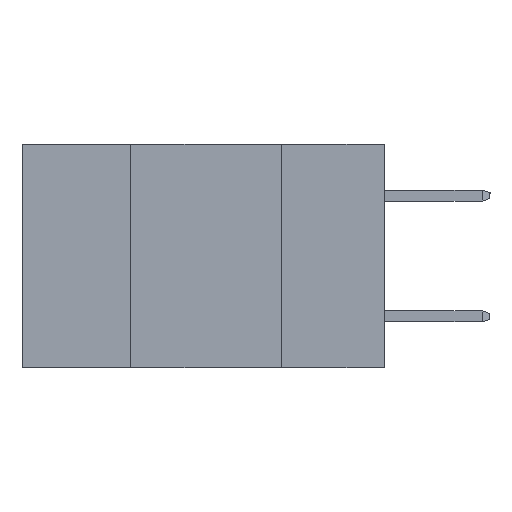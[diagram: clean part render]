
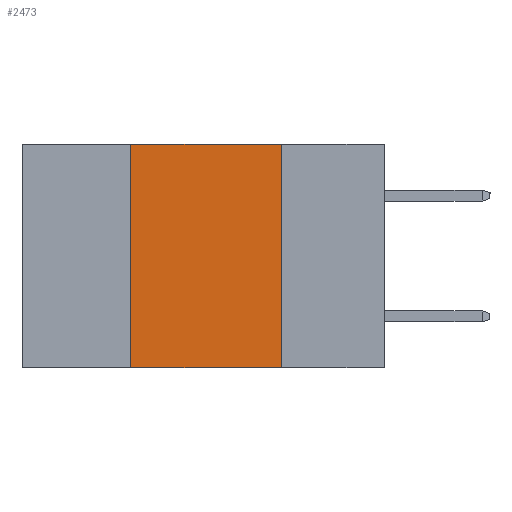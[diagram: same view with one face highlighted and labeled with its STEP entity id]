
A CAD part, left-side view. The second image highlights one B-rep face of the part: STEP entity #2473.
In plain terms, the highlighted planar face has unit normal (-1, 0, 0).
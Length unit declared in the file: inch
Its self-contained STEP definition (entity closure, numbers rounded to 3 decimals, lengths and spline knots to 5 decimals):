
#1633 = VECTOR ( 'NONE', #8139, 39.37008 ) ;
#2008 = ORIENTED_EDGE ( 'NONE', *, *, #7815, .F. ) ;
#2473 = ADVANCED_FACE ( 'NONE', ( #11334 ), #6077, .F. ) ;
#3653 = VECTOR ( 'NONE', #16933, 39.37008 ) ;
#3939 = ORIENTED_EDGE ( 'NONE', *, *, #19292, .F. ) ;
#4271 = EDGE_CURVE ( 'NONE', #17961, #8135, #6595, .T. ) ;
#4904 = EDGE_LOOP ( 'NONE', ( #3939, #17289, #2008, #9329 ) ) ;
#6077 = PLANE ( 'NONE',  #19034 ) ;
#6259 = VECTOR ( 'NONE', #8287, 39.37008 ) ;
#6595 = LINE ( 'NONE', #10071, #6259 ) ;
#6774 = LINE ( 'NONE', #18643, #1633 ) ;
#7815 = EDGE_CURVE ( 'NONE', #17961, #15126, #6774, .T. ) ;
#8135 = VERTEX_POINT ( 'NONE', #19822 ) ;
#8139 = DIRECTION ( 'NONE',  ( 0., 0., 1. ) ) ;
#8287 = DIRECTION ( 'NONE',  ( 0., -1., 0. ) ) ;
#9329 = ORIENTED_EDGE ( 'NONE', *, *, #4271, .T. ) ;
#9493 = VECTOR ( 'NONE', #20148, 39.37008 ) ;
#10071 = CARTESIAN_POINT ( 'NONE',  ( 0., 0.6, -0.37 ) ) ;
#11334 = FACE_OUTER_BOUND ( 'NONE', #4904, .T. ) ;
#11854 = VERTEX_POINT ( 'NONE', #12383 ) ;
#11885 = LINE ( 'NONE', #22098, #3653 ) ;
#12383 = CARTESIAN_POINT ( 'NONE',  ( 0., 0.17, 0. ) ) ;
#13191 = CARTESIAN_POINT ( 'NONE',  ( 0., 0.17, -0.37 ) ) ;
#13498 = EDGE_CURVE ( 'NONE', #15126, #11854, #11885, .T. ) ;
#13590 = CARTESIAN_POINT ( 'NONE',  ( 0., 0.42, -0.37 ) ) ;
#15017 = DIRECTION ( 'NONE',  ( 0., 0., -1. ) ) ;
#15126 = VERTEX_POINT ( 'NONE', #15603 ) ;
#15603 = CARTESIAN_POINT ( 'NONE',  ( 0., 0.42, 0. ) ) ;
#16480 = CARTESIAN_POINT ( 'NONE',  ( 0., 0.6, 0. ) ) ;
#16933 = DIRECTION ( 'NONE',  ( 0., -1., 0. ) ) ;
#17289 = ORIENTED_EDGE ( 'NONE', *, *, #13498, .F. ) ;
#17961 = VERTEX_POINT ( 'NONE', #13590 ) ;
#18463 = LINE ( 'NONE', #13191, #9493 ) ;
#18643 = CARTESIAN_POINT ( 'NONE',  ( 0., 0.42, -0.37 ) ) ;
#19034 = AXIS2_PLACEMENT_3D ( 'NONE', #16480, #21758, #15017 ) ;
#19292 = EDGE_CURVE ( 'NONE', #11854, #8135, #18463, .T. ) ;
#19822 = CARTESIAN_POINT ( 'NONE',  ( 0., 0.17, -0.37 ) ) ;
#20148 = DIRECTION ( 'NONE',  ( 0., 0., -1. ) ) ;
#21758 = DIRECTION ( 'NONE',  ( 1., 0., 0. ) ) ;
#22098 = CARTESIAN_POINT ( 'NONE',  ( 0., 0.6, 0. ) ) ;
